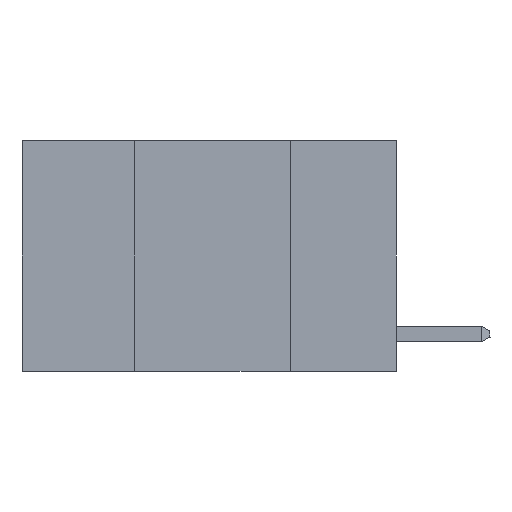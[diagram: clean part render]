
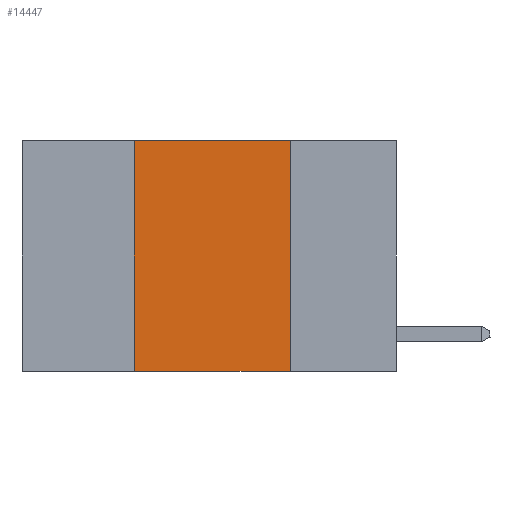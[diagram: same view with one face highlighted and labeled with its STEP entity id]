
A CAD part, left-side view. The second image highlights one B-rep face of the part: STEP entity #14447.
In plain terms, the highlighted planar face has unit normal (-1, 0, 0).
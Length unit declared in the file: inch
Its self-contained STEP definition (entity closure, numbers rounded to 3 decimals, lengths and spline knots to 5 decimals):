
#67 = EDGE_CURVE ( 'NONE', #21372, #23739, #24894, .T. ) ;
#422 = ORIENTED_EDGE ( 'NONE', *, *, #15973, .F. ) ;
#2958 = CARTESIAN_POINT ( 'NONE',  ( 0., 0.17, 0. ) ) ;
#3120 = CARTESIAN_POINT ( 'NONE',  ( 0., 0.42, -0.37 ) ) ;
#3319 = LINE ( 'NONE', #13538, #13814 ) ;
#4997 = ORIENTED_EDGE ( 'NONE', *, *, #7066, .F. ) ;
#5593 = CARTESIAN_POINT ( 'NONE',  ( 0., 0.42, 0. ) ) ;
#6784 = EDGE_CURVE ( 'NONE', #21372, #9844, #15397, .T. ) ;
#7066 = EDGE_CURVE ( 'NONE', #20328, #23739, #11147, .T. ) ;
#7400 = ORIENTED_EDGE ( 'NONE', *, *, #6784, .F. ) ;
#7473 = DIRECTION ( 'NONE',  ( 0., -1., 0. ) ) ;
#9421 = DIRECTION ( 'NONE',  ( 0., 0., -1. ) ) ;
#9844 = VERTEX_POINT ( 'NONE', #19358 ) ;
#10771 = CARTESIAN_POINT ( 'NONE',  ( 0., 0.17, -0.37 ) ) ;
#11147 = LINE ( 'NONE', #2958, #23329 ) ;
#11195 = FACE_OUTER_BOUND ( 'NONE', #14996, .T. ) ;
#11588 = PLANE ( 'NONE',  #20708 ) ;
#12511 = ORIENTED_EDGE ( 'NONE', *, *, #67, .T. ) ;
#12680 = VECTOR ( 'NONE', #21242, 39.37008 ) ;
#13149 = DIRECTION ( 'NONE',  ( 0., -1., 0. ) ) ;
#13538 = CARTESIAN_POINT ( 'NONE',  ( 0., 0.6, 0. ) ) ;
#13814 = VECTOR ( 'NONE', #13149, 39.37008 ) ;
#13926 = CARTESIAN_POINT ( 'NONE',  ( 0., 0.17, 0. ) ) ;
#14447 = ADVANCED_FACE ( 'NONE', ( #11195 ), #11588, .F. ) ;
#14996 = EDGE_LOOP ( 'NONE', ( #4997, #422, #7400, #12511 ) ) ;
#15397 = LINE ( 'NONE', #5593, #12680 ) ;
#15973 = EDGE_CURVE ( 'NONE', #9844, #20328, #3319, .T. ) ;
#16862 = DIRECTION ( 'NONE',  ( 0., 0., -1. ) ) ;
#17168 = DIRECTION ( 'NONE',  ( 1., 0., 0. ) ) ;
#17513 = CARTESIAN_POINT ( 'NONE',  ( 0., 0.6, -0.37 ) ) ;
#19358 = CARTESIAN_POINT ( 'NONE',  ( 0., 0.42, 0. ) ) ;
#20328 = VERTEX_POINT ( 'NONE', #13926 ) ;
#20708 = AXIS2_PLACEMENT_3D ( 'NONE', #20827, #17168, #9421 ) ;
#20827 = CARTESIAN_POINT ( 'NONE',  ( 0., 0.6, 0. ) ) ;
#21242 = DIRECTION ( 'NONE',  ( 0., 0., 1. ) ) ;
#21372 = VERTEX_POINT ( 'NONE', #3120 ) ;
#21779 = VECTOR ( 'NONE', #7473, 39.37008 ) ;
#23329 = VECTOR ( 'NONE', #16862, 39.37008 ) ;
#23739 = VERTEX_POINT ( 'NONE', #10771 ) ;
#24894 = LINE ( 'NONE', #17513, #21779 ) ;
